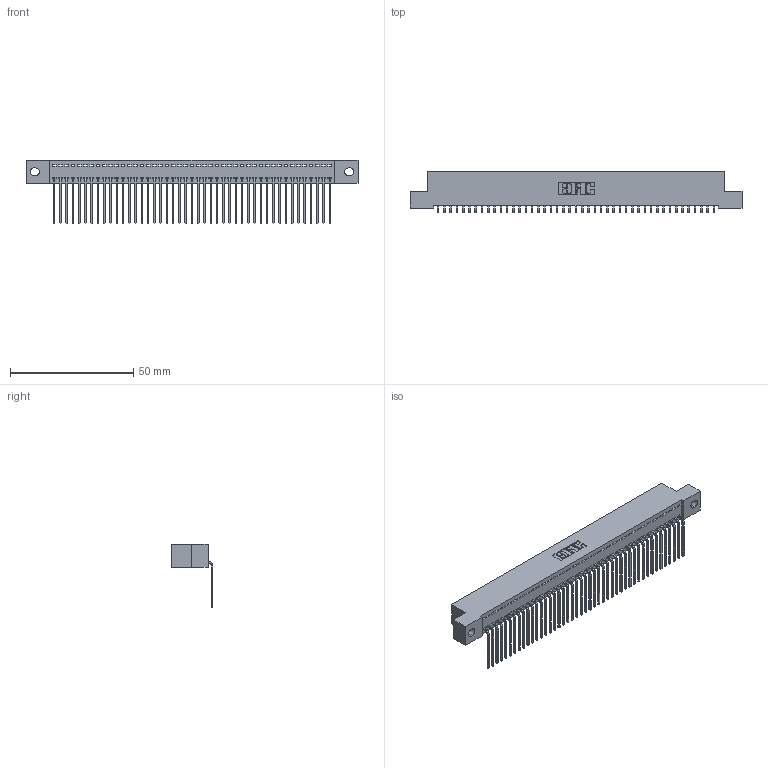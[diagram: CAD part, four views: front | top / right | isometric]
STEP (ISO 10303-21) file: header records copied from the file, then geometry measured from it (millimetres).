
FILE_DESCRIPTION (( 'STEP AP203' ), '1' );
FILE_NAME ('342-045-559-102.STEP', '2019-10-02T20:05:14', ( '' ), ( '' ), 'SwSTEP 2.0', 'SolidWorks 2016', '' );
FILE_SCHEMA (( 'CONFIG_CONTROL_DESIGN' ));
Length unit declared in the file: inch
Products named in the file (3): 342 Part_.128 Slot; 345-292-001_558 559 Tail - 1; 342-045-559-102
Assembly tree (46 placements, depth 2):
  342-045-559-102
    342 Part_.128 Slot
    345-292-001_558 559 Tail - 1  x45
Bounding box: 134.62 x 16.83 x 25.78 mm (x, y, z)
Volume: 11912.3 mm3; surface area: 18159.8 mm2
Topology: 46 solids, 46 shells, 2814 faces, 8501 edges, 5606 vertices
Faces by surface type: plane 2050, cylinder 764
Entity records: 27209 total; most frequent: CARTESIAN_POINT 4701, ORIENTED_EDGE 4682, DIRECTION 3959, EDGE_CURVE 2341, VECTOR 2213, LINE 2213, VERTEX_POINT 1558, AXIS2_PLACEMENT_3D 873
